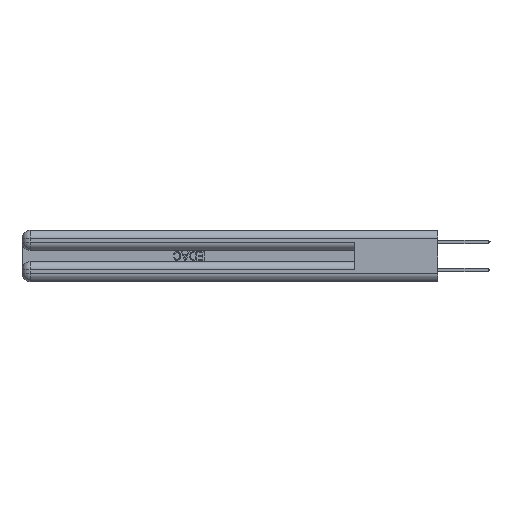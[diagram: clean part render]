
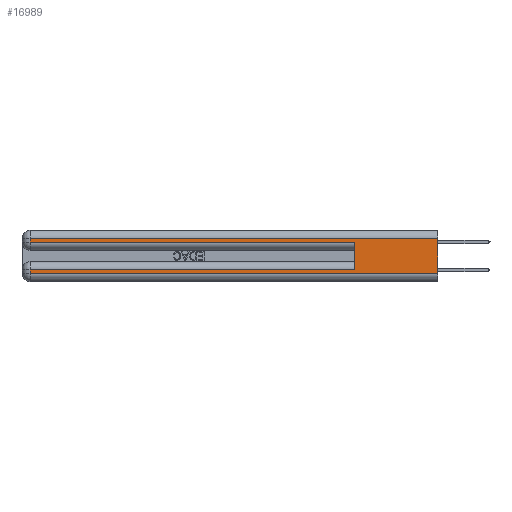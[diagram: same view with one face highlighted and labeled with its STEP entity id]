
A CAD part, left-side view. The second image highlights one B-rep face of the part: STEP entity #16989.
In plain terms, the highlighted planar face has unit normal (-1, 0, 0).
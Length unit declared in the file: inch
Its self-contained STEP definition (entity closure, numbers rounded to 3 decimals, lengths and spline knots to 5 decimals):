
#218 = ORIENTED_EDGE ( 'NONE', *, *, #35631, .T. ) ;
#690 = CARTESIAN_POINT ( 'NONE',  ( 0., 0., 0.31 ) ) ;
#793 = EDGE_CURVE ( 'NONE', #21952, #9101, #8816, .T. ) ;
#958 = LINE ( 'NONE', #4217, #37640 ) ;
#1633 = DIRECTION ( 'NONE',  ( 0., -1., 0. ) ) ;
#1761 = EDGE_CURVE ( 'NONE', #19833, #31485, #31622, .T. ) ;
#2518 = DIRECTION ( 'NONE',  ( 0., 0., -1. ) ) ;
#2832 = LINE ( 'NONE', #33334, #37527 ) ;
#3569 = VECTOR ( 'NONE', #35200, 39.37008 ) ;
#4201 = ORIENTED_EDGE ( 'NONE', *, *, #25795, .F. ) ;
#4217 = CARTESIAN_POINT ( 'NONE',  ( 0., 0., 0.31 ) ) ;
#5410 = CARTESIAN_POINT ( 'NONE',  ( 0., 0., 0.37 ) ) ;
#7789 = LINE ( 'NONE', #15192, #9681 ) ;
#8816 = LINE ( 'NONE', #34904, #24468 ) ;
#9101 = VERTEX_POINT ( 'NONE', #26237 ) ;
#9149 = CARTESIAN_POINT ( 'NONE',  ( 0., 2.94, 0.31 ) ) ;
#9681 = VECTOR ( 'NONE', #23959, 39.37008 ) ;
#9755 = VERTEX_POINT ( 'NONE', #24525 ) ;
#11102 = EDGE_CURVE ( 'NONE', #12435, #31857, #958, .T. ) ;
#11570 = VECTOR ( 'NONE', #14588, 39.37008 ) ;
#11651 = DIRECTION ( 'NONE',  ( 1., 0., 0. ) ) ;
#11928 = ORIENTED_EDGE ( 'NONE', *, *, #1761, .F. ) ;
#12435 = VERTEX_POINT ( 'NONE', #690 ) ;
#13583 = CARTESIAN_POINT ( 'NONE',  ( 0., 0., 0.085 ) ) ;
#13631 = DIRECTION ( 'NONE',  ( 0., 1., 0. ) ) ;
#14588 = DIRECTION ( 'NONE',  ( 0., 0., -1. ) ) ;
#15192 = CARTESIAN_POINT ( 'NONE',  ( 0., 0., 0.37 ) ) ;
#15960 = ORIENTED_EDGE ( 'NONE', *, *, #26764, .T. ) ;
#16989 = ADVANCED_FACE ( 'NONE', ( #24088 ), #20642, .F. ) ;
#17032 = DIRECTION ( 'NONE',  ( 0., -1., 0. ) ) ;
#17078 = CARTESIAN_POINT ( 'NONE',  ( 0., 2.94, 0.06 ) ) ;
#18372 = DIRECTION ( 'NONE',  ( 0., 0., -1. ) ) ;
#19577 = LINE ( 'NONE', #36070, #11570 ) ;
#19675 = LINE ( 'NONE', #13583, #3569 ) ;
#19833 = VERTEX_POINT ( 'NONE', #38458 ) ;
#20542 = VERTEX_POINT ( 'NONE', #25507 ) ;
#20642 = PLANE ( 'NONE',  #39155 ) ;
#21069 = LINE ( 'NONE', #32352, #25311 ) ;
#21158 = ORIENTED_EDGE ( 'NONE', *, *, #37103, .T. ) ;
#21952 = VERTEX_POINT ( 'NONE', #17078 ) ;
#23451 = ORIENTED_EDGE ( 'NONE', *, *, #793, .T. ) ;
#23490 = VECTOR ( 'NONE', #39257, 39.37008 ) ;
#23959 = DIRECTION ( 'NONE',  ( 0., 0., -1. ) ) ;
#24088 = FACE_OUTER_BOUND ( 'NONE', #29013, .T. ) ;
#24468 = VECTOR ( 'NONE', #1633, 39.37008 ) ;
#24525 = CARTESIAN_POINT ( 'NONE',  ( 0., 2.94, 0.285 ) ) ;
#25311 = VECTOR ( 'NONE', #17032, 39.37008 ) ;
#25507 = CARTESIAN_POINT ( 'NONE',  ( 0., 2.94, 0.085 ) ) ;
#25795 = EDGE_CURVE ( 'NONE', #12435, #9101, #7789, .T. ) ;
#26237 = CARTESIAN_POINT ( 'NONE',  ( 0., 0., 0.06 ) ) ;
#26764 = EDGE_CURVE ( 'NONE', #9755, #31485, #21069, .T. ) ;
#29013 = EDGE_LOOP ( 'NONE', ( #4201, #34981, #21158, #15960, #11928, #218, #34398, #23451 ) ) ;
#29015 = CARTESIAN_POINT ( 'NONE',  ( 0., 0.6, 0.285 ) ) ;
#31485 = VERTEX_POINT ( 'NONE', #29015 ) ;
#31622 = LINE ( 'NONE', #39385, #23490 ) ;
#31857 = VERTEX_POINT ( 'NONE', #9149 ) ;
#32352 = CARTESIAN_POINT ( 'NONE',  ( 0., 0., 0.285 ) ) ;
#33334 = CARTESIAN_POINT ( 'NONE',  ( 0., 2.94, 0.37 ) ) ;
#33696 = EDGE_CURVE ( 'NONE', #20542, #21952, #2832, .T. ) ;
#34398 = ORIENTED_EDGE ( 'NONE', *, *, #33696, .T. ) ;
#34904 = CARTESIAN_POINT ( 'NONE',  ( 0., 0., 0.06 ) ) ;
#34981 = ORIENTED_EDGE ( 'NONE', *, *, #11102, .T. ) ;
#35200 = DIRECTION ( 'NONE',  ( 0., 1., 0. ) ) ;
#35631 = EDGE_CURVE ( 'NONE', #19833, #20542, #19675, .T. ) ;
#36070 = CARTESIAN_POINT ( 'NONE',  ( 0., 2.94, 0.37 ) ) ;
#37103 = EDGE_CURVE ( 'NONE', #31857, #9755, #19577, .T. ) ;
#37527 = VECTOR ( 'NONE', #18372, 39.37008 ) ;
#37640 = VECTOR ( 'NONE', #13631, 39.37008 ) ;
#38458 = CARTESIAN_POINT ( 'NONE',  ( 0., 0.6, 0.085 ) ) ;
#39155 = AXIS2_PLACEMENT_3D ( 'NONE', #5410, #11651, #2518 ) ;
#39257 = DIRECTION ( 'NONE',  ( 0., 0., 1. ) ) ;
#39385 = CARTESIAN_POINT ( 'NONE',  ( 0., 0.6, 0.145 ) ) ;
